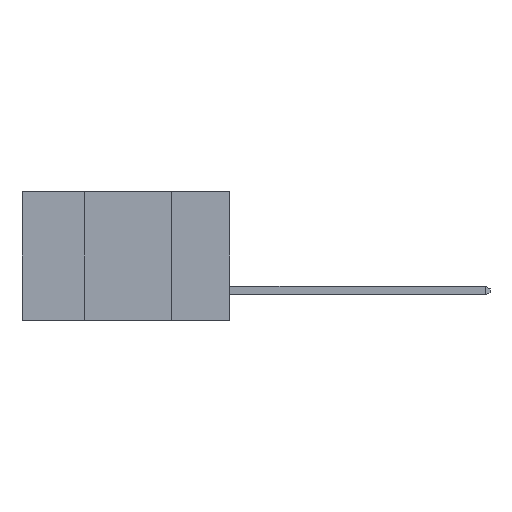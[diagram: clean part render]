
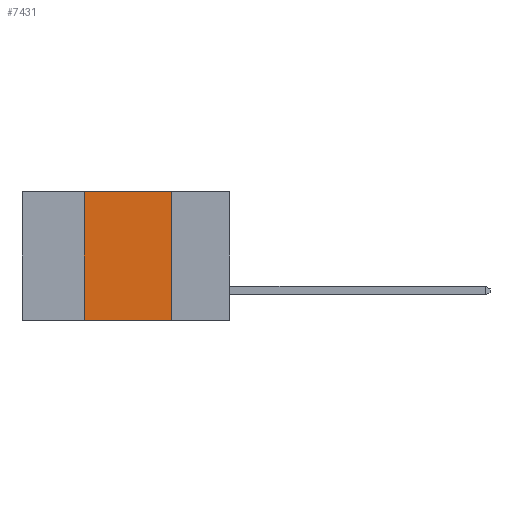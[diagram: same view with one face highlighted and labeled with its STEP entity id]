
A CAD part, left-side view. The second image highlights one B-rep face of the part: STEP entity #7431.
In plain terms, the highlighted planar face has unit normal (-1, 0, 0).
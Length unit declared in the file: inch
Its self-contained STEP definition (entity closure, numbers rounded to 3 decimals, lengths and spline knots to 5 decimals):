
#31 = DIRECTION ( 'NONE',  ( 0., 0., -1. ) ) ;
#433 = FACE_OUTER_BOUND ( 'NONE', #11182, .T. ) ;
#668 = CARTESIAN_POINT ( 'NONE',  ( 0., 0.6, 0. ) ) ;
#1628 = DIRECTION ( 'NONE',  ( 0., 0., 1. ) ) ;
#2078 = CARTESIAN_POINT ( 'NONE',  ( 0., 0.42, -0.37 ) ) ;
#2179 = VERTEX_POINT ( 'NONE', #8695 ) ;
#2886 = LINE ( 'NONE', #2078, #13062 ) ;
#2893 = CARTESIAN_POINT ( 'NONE',  ( 0., 0.42, 0. ) ) ;
#3789 = EDGE_CURVE ( 'NONE', #2179, #8273, #10729, .T. ) ;
#4781 = VERTEX_POINT ( 'NONE', #5113 ) ;
#4782 = LINE ( 'NONE', #12878, #13001 ) ;
#4796 = VECTOR ( 'NONE', #31, 39.37008 ) ;
#4951 = DIRECTION ( 'NONE',  ( 1., 0., 0. ) ) ;
#5113 = CARTESIAN_POINT ( 'NONE',  ( 0., 0.42, -0.37 ) ) ;
#7212 = ORIENTED_EDGE ( 'NONE', *, *, #11104, .T. ) ;
#7406 = CARTESIAN_POINT ( 'NONE',  ( 0., 0.17, -0.37 ) ) ;
#7431 = ADVANCED_FACE ( 'NONE', ( #433 ), #11246, .F. ) ;
#8273 = VERTEX_POINT ( 'NONE', #7406 ) ;
#8695 = CARTESIAN_POINT ( 'NONE',  ( 0., 0.17, 0. ) ) ;
#8747 = DIRECTION ( 'NONE',  ( 0., -1., 0. ) ) ;
#9059 = VERTEX_POINT ( 'NONE', #2893 ) ;
#9257 = EDGE_CURVE ( 'NONE', #4781, #9059, #2886, .T. ) ;
#9494 = ORIENTED_EDGE ( 'NONE', *, *, #9257, .F. ) ;
#9759 = EDGE_CURVE ( 'NONE', #9059, #2179, #11232, .T. ) ;
#10485 = DIRECTION ( 'NONE',  ( 0., -1., 0. ) ) ;
#10729 = LINE ( 'NONE', #12468, #4796 ) ;
#11104 = EDGE_CURVE ( 'NONE', #4781, #8273, #4782, .T. ) ;
#11182 = EDGE_LOOP ( 'NONE', ( #13289, #11793, #9494, #7212 ) ) ;
#11232 = LINE ( 'NONE', #11458, #13363 ) ;
#11246 = PLANE ( 'NONE',  #13028 ) ;
#11458 = CARTESIAN_POINT ( 'NONE',  ( 0., 0.6, 0. ) ) ;
#11793 = ORIENTED_EDGE ( 'NONE', *, *, #9759, .F. ) ;
#12468 = CARTESIAN_POINT ( 'NONE',  ( 0., 0.17, -0.37 ) ) ;
#12878 = CARTESIAN_POINT ( 'NONE',  ( 0., 0.6, -0.37 ) ) ;
#13001 = VECTOR ( 'NONE', #8747, 39.37008 ) ;
#13028 = AXIS2_PLACEMENT_3D ( 'NONE', #668, #4951, #13172 ) ;
#13062 = VECTOR ( 'NONE', #1628, 39.37008 ) ;
#13172 = DIRECTION ( 'NONE',  ( 0., 0., -1. ) ) ;
#13289 = ORIENTED_EDGE ( 'NONE', *, *, #3789, .F. ) ;
#13363 = VECTOR ( 'NONE', #10485, 39.37008 ) ;
